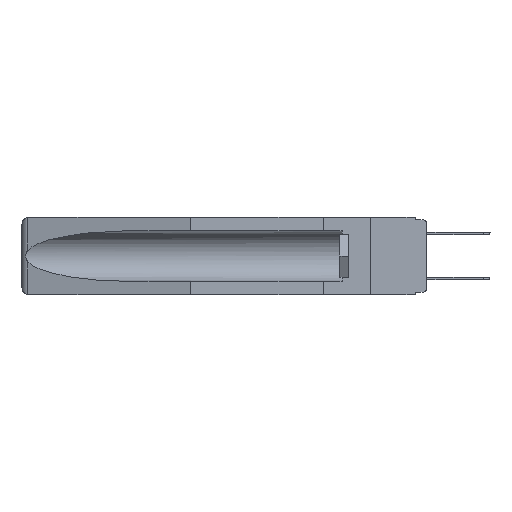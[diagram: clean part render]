
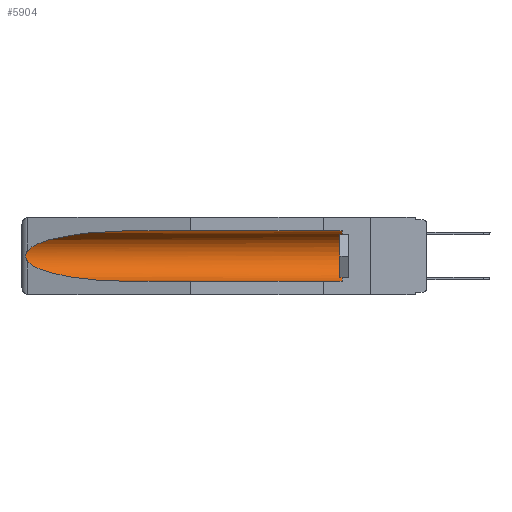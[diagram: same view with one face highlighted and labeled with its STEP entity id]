
A CAD part, left-side view. The second image highlights one B-rep face of the part: STEP entity #5904.
In plain terms, the highlighted cylindrical face has radius 2.857 mm (diameter 5.715 mm), a partial arc.
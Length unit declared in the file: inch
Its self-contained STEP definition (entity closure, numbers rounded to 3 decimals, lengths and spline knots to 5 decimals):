
#485 = EDGE_CURVE ( 'NONE', #3944, #5580, #4865, .T. ) ;
#653 = EDGE_CURVE ( 'NONE', #14869, #14424, #14129, .T. ) ;
#671 = CARTESIAN_POINT ( 'NONE',  ( 0.21114, 1.30732, -0.059 ) ) ;
#840 = ORIENTED_EDGE ( 'NONE', *, *, #653, .T. ) ;
#1323 = CARTESIAN_POINT ( 'NONE',  ( 0.26654, 1.53092, -0.15636 ) ) ;
#1407 = CARTESIAN_POINT ( 'NONE',  ( 0.155, -0.30754, -0.1715 ) ) ;
#1854 = CARTESIAN_POINT ( 'NONE',  ( 0.155, 1.07973, -0.059 ) ) ;
#2581 = CARTESIAN_POINT ( 'NONE',  ( 0.155, 1.07973, -0.059 ) ) ;
#2759 = CARTESIAN_POINT ( 'NONE',  ( 0.26537, 1.52718, -0.19328 ) ) ;
#2777 = CARTESIAN_POINT ( 'NONE',  ( 0.155, 1.07973, -0.284 ) ) ;
#3024 = ORIENTED_EDGE ( 'NONE', *, *, #11775, .T. ) ;
#3164 = CARTESIAN_POINT ( 'NONE',  ( 0.155, 0.126, -0.284 ) ) ;
#3878 = FACE_OUTER_BOUND ( 'NONE', #11962, .T. ) ;
#3944 = VERTEX_POINT ( 'NONE', #3164 ) ;
#4865 = LINE ( 'NONE', #11585, #16002 ) ;
#5280 = VECTOR ( 'NONE', #21019, 39.37008 ) ;
#5580 = VERTEX_POINT ( 'NONE', #2777 ) ;
#5904 = ADVANCED_FACE ( 'NONE', ( #3878 ), #7346, .F. ) ;
#5964 = EDGE_CURVE ( 'NONE', #12312, #5580, #20214, .T. ) ;
#6231 = DIRECTION ( 'NONE',  ( 0., 0., 1. ) ) ;
#6483 = CARTESIAN_POINT ( 'NONE',  ( 0.26597, 1.5296, -0.19026 ) ) ;
#6568 = DIRECTION ( 'NONE',  ( 0., 1., 0. ) ) ;
#7346 = CYLINDRICAL_SURFACE ( 'NONE', #14701, 0.1125 ) ;
#7818 = DIRECTION ( 'NONE',  ( 0., -1., 0. ) ) ;
#8149 = CARTESIAN_POINT ( 'NONE',  ( 0.2673, 1.5327, -0.16383 ) ) ;
#8539 = CARTESIAN_POINT ( 'NONE',  ( 0.155, 0.126, -0.059 ) ) ;
#8717 = EDGE_CURVE ( 'NONE', #9167, #12312, #10893, .T. ) ;
#8737 = AXIS2_PLACEMENT_3D ( 'NONE', #16352, #7818, #14641 ) ;
#9167 = VERTEX_POINT ( 'NONE', #16534 ) ;
#9388 = ORIENTED_EDGE ( 'NONE', *, *, #485, .F. ) ;
#9565 = CARTESIAN_POINT ( 'NONE',  ( 0.25451, 1.48313, -0.24835 ) ) ;
#10008 = EDGE_CURVE ( 'NONE', #14424, #9167, #18089, .T. ) ;
#10281 = CARTESIAN_POINT ( 'NONE',  ( 0.2675, 1.53308, -0.17534 ) ) ;
#10578 = ORIENTED_EDGE ( 'NONE', *, *, #5964, .T. ) ;
#10874 = CARTESIAN_POINT ( 'NONE',  ( 0.25451, 1.48313, -0.09465 ) ) ;
#10893 = B_SPLINE_CURVE_WITH_KNOTS ( 'NONE', 3,
 ( #16685, #21520, #1323, #8149, #21855, #10281, #16792, #13292, #6483, #18709 ),
 .UNSPECIFIED., .F., .F.,
 ( 4, 2, 2, 2, 4 ),
 ( 0., 0.00029, 0.00058, 0.00087, 0.00117 ),
 .UNSPECIFIED. ) ;
#11266 = CARTESIAN_POINT ( 'NONE',  ( 0.155, 1.07973, -0.284 ) ) ;
#11315 = CARTESIAN_POINT ( 'NONE',  ( 0.26537, 1.52718, -0.14972 ) ) ;
#11585 = CARTESIAN_POINT ( 'NONE',  ( 0.155, -0.30754, -0.284 ) ) ;
#11775 = EDGE_CURVE ( 'NONE', #3944, #14869, #17697, .T. ) ;
#11962 = EDGE_LOOP ( 'NONE', ( #21165, #15164, #10578, #9388, #3024, #840 ) ) ;
#12312 = VERTEX_POINT ( 'NONE', #2759 ) ;
#13151 = CARTESIAN_POINT ( 'NONE',  ( 0.21114, 1.30732, -0.284 ) ) ;
#13292 = CARTESIAN_POINT ( 'NONE',  ( 0.26655, 1.53094, -0.18657 ) ) ;
#14129 = LINE ( 'NONE', #17625, #5280 ) ;
#14424 = VERTEX_POINT ( 'NONE', #1854 ) ;
#14641 = DIRECTION ( 'NONE',  ( 0., 0., 1. ) ) ;
#14701 = AXIS2_PLACEMENT_3D ( 'NONE', #1407, #6568, #6231 ) ;
#14869 = VERTEX_POINT ( 'NONE', #8539 ) ;
#15164 = ORIENTED_EDGE ( 'NONE', *, *, #8717, .T. ) ;
#16002 = VECTOR ( 'NONE', #17085, 39.37008 ) ;
#16352 = CARTESIAN_POINT ( 'NONE',  ( 0.155, 0.126, -0.1715 ) ) ;
#16534 = CARTESIAN_POINT ( 'NONE',  ( 0.26537, 1.52718, -0.14972 ) ) ;
#16685 = CARTESIAN_POINT ( 'NONE',  ( 0.26537, 1.52718, -0.14972 ) ) ;
#16792 = CARTESIAN_POINT ( 'NONE',  ( 0.2673, 1.53269, -0.17917 ) ) ;
#17085 = DIRECTION ( 'NONE',  ( 0., 1., 0. ) ) ;
#17625 = CARTESIAN_POINT ( 'NONE',  ( 0.155, -0.30754, -0.059 ) ) ;
#17697 = CIRCLE ( 'NONE', #8737, 0.1125 ) ;
#18089 =( BOUNDED_CURVE ( )  B_SPLINE_CURVE ( 3, ( #2581, #671, #10874, #11315 ),
 .UNSPECIFIED., .F., .F. ) 
 B_SPLINE_CURVE_WITH_KNOTS ( ( 4, 4 ),
 ( 4.71239, 6.08839 ),
 .UNSPECIFIED. ) 
 CURVE ( )  GEOMETRIC_REPRESENTATION_ITEM ( )  RATIONAL_B_SPLINE_CURVE ( ( 1., 0.848, 0.848, 1. ) ) 
 REPRESENTATION_ITEM ( '' )  );
#18709 = CARTESIAN_POINT ( 'NONE',  ( 0.26537, 1.52718, -0.19328 ) ) ;
#19798 = CARTESIAN_POINT ( 'NONE',  ( 0.26537, 1.52718, -0.19328 ) ) ;
#20214 =( BOUNDED_CURVE ( )  B_SPLINE_CURVE ( 3, ( #19798, #9565, #13151, #11266 ),
 .UNSPECIFIED., .F., .F. ) 
 B_SPLINE_CURVE_WITH_KNOTS ( ( 4, 4 ),
 ( 0.1948, 1.5708 ),
 .UNSPECIFIED. ) 
 CURVE ( )  GEOMETRIC_REPRESENTATION_ITEM ( )  RATIONAL_B_SPLINE_CURVE ( ( 1., 0.848, 0.848, 1. ) ) 
 REPRESENTATION_ITEM ( '' )  );
#21019 = DIRECTION ( 'NONE',  ( 0., 1., 0. ) ) ;
#21165 = ORIENTED_EDGE ( 'NONE', *, *, #10008, .T. ) ;
#21520 = CARTESIAN_POINT ( 'NONE',  ( 0.26597, 1.52961, -0.15275 ) ) ;
#21855 = CARTESIAN_POINT ( 'NONE',  ( 0.2675, 1.53308, -0.16763 ) ) ;
